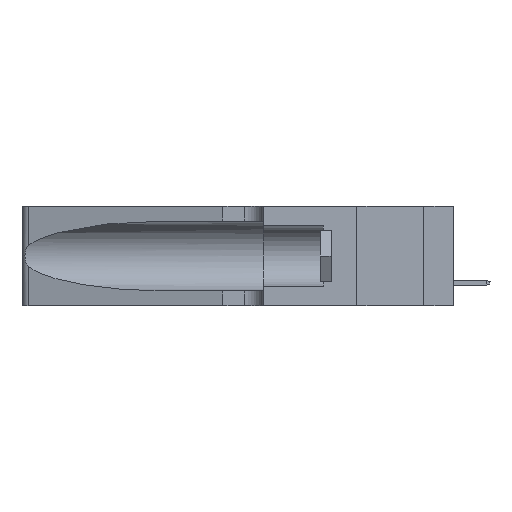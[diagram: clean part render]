
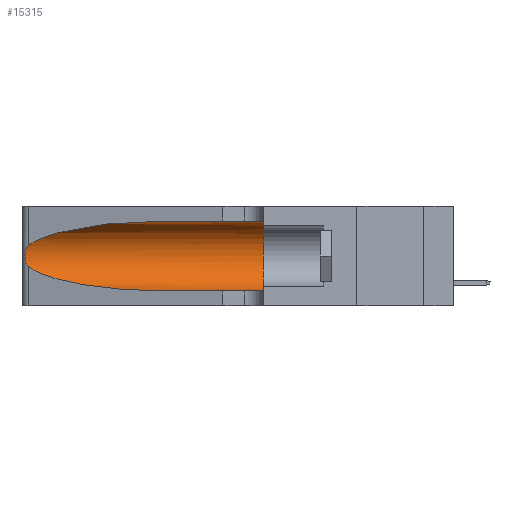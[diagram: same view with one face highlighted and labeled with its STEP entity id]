
A CAD part, left-side view. The second image highlights one B-rep face of the part: STEP entity #15315.
In plain terms, the highlighted cylindrical face has radius 3.308 mm (diameter 6.617 mm), a partial arc.
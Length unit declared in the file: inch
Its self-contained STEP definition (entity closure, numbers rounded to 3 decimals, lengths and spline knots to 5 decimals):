
#363 = EDGE_CURVE ( 'NONE', #2878, #23513, #11433, .T. ) ;
#1574 = CARTESIAN_POINT ( 'NONE',  ( 0.25856, 1.23593, 0.16098 ) ) ;
#1844 = VERTEX_POINT ( 'NONE', #21979 ) ;
#2344 = DIRECTION ( 'NONE',  ( 0., 1., 0. ) ) ;
#2723 = VERTEX_POINT ( 'NONE', #18269 ) ;
#2774 = CARTESIAN_POINT ( 'NONE',  ( 0.1305, 0.35, 0.185 ) ) ;
#2878 = VERTEX_POINT ( 'NONE', #11497 ) ;
#3620 = EDGE_CURVE ( 'NONE', #1844, #23513, #6035, .T. ) ;
#3832 = CARTESIAN_POINT ( 'NONE',  ( 0.25787, 1.23484, 0.2124 ) ) ;
#3941 = VERTEX_POINT ( 'NONE', #9408 ) ;
#4135 = ORIENTED_EDGE ( 'NONE', *, *, #26418, .T. ) ;
#4533 = LINE ( 'NONE', #20291, #17077 ) ;
#4719 = VERTEX_POINT ( 'NONE', #18321 ) ;
#4834 =( BOUNDED_CURVE ( )  B_SPLINE_CURVE ( 3, ( #23729, #9476, #16378, #16237 ),
 .UNSPECIFIED., .F., .T. ) 
 B_SPLINE_CURVE_WITH_KNOTS ( ( 4, 4 ),
 ( 1.5708, 2.84003 ),
 .UNSPECIFIED. ) 
 CURVE ( )  GEOMETRIC_REPRESENTATION_ITEM ( )  RATIONAL_B_SPLINE_CURVE ( ( 1., 0.87, 0.87, 1. ) ) 
 REPRESENTATION_ITEM ( '' )  );
#6035 = LINE ( 'NONE', #15182, #9182 ) ;
#6378 = CARTESIAN_POINT ( 'NONE',  ( 0.25487, 1.22718, 0.14631 ) ) ;
#6846 = EDGE_LOOP ( 'NONE', ( #17508, #28582, #4135, #7560, #24842, #8613 ) ) ;
#7560 = ORIENTED_EDGE ( 'NONE', *, *, #3620, .T. ) ;
#7723 = DIRECTION ( 'NONE',  ( 0., 0., -1. ) ) ;
#8321 = CARTESIAN_POINT ( 'NONE',  ( 0.26075, 1.23896, 0.178 ) ) ;
#8613 = ORIENTED_EDGE ( 'NONE', *, *, #19856, .F. ) ;
#8616 = CARTESIAN_POINT ( 'NONE',  ( 0.26017, 1.23833, 0.17102 ) ) ;
#9182 = VECTOR ( 'NONE', #24656, 39.37008 ) ;
#9408 = CARTESIAN_POINT ( 'NONE',  ( 0.25487, 1.22718, 0.22369 ) ) ;
#9476 = CARTESIAN_POINT ( 'NONE',  ( 0.18966, 0.96281, 0.31525 ) ) ;
#9521 = DIRECTION ( 'NONE',  ( 0., 0., 1. ) ) ;
#9732 = AXIS2_PLACEMENT_3D ( 'NONE', #21690, #19577, #7723 ) ;
#10725 = CARTESIAN_POINT ( 'NONE',  ( 0.25555, 1.22993, 0.14849 ) ) ;
#10987 = CARTESIAN_POINT ( 'NONE',  ( 0.18966, 0.96281, 0.05475 ) ) ;
#11289 = CARTESIAN_POINT ( 'NONE',  ( 0.25487, 1.22718, 0.14631 ) ) ;
#11433 = CIRCLE ( 'NONE', #21479, 0.13025 ) ;
#11497 = CARTESIAN_POINT ( 'NONE',  ( 0.1305, 0.35, 0.31525 ) ) ;
#12967 = CARTESIAN_POINT ( 'NONE',  ( 0.26075, 1.23896, 0.19203 ) ) ;
#13117 = CARTESIAN_POINT ( 'NONE',  ( 0.25854, 1.2359, 0.20912 ) ) ;
#13267 = CARTESIAN_POINT ( 'NONE',  ( 0.26018, 1.23835, 0.19895 ) ) ;
#13670 = DIRECTION ( 'NONE',  ( 0., -1., 0. ) ) ;
#14471 = FACE_OUTER_BOUND ( 'NONE', #6846, .T. ) ;
#14772 = CYLINDRICAL_SURFACE ( 'NONE', #9732, 0.13025 ) ;
#14998 =( BOUNDED_CURVE ( )  B_SPLINE_CURVE ( 3, ( #11289, #25112, #10987, #20154 ),
 .UNSPECIFIED., .F., .T. ) 
 B_SPLINE_CURVE_WITH_KNOTS ( ( 4, 4 ),
 ( 3.44316, 4.71239 ),
 .UNSPECIFIED. ) 
 CURVE ( )  GEOMETRIC_REPRESENTATION_ITEM ( )  RATIONAL_B_SPLINE_CURVE ( ( 1., 0.87, 0.87, 1. ) ) 
 REPRESENTATION_ITEM ( '' )  );
#15182 = CARTESIAN_POINT ( 'NONE',  ( 0.1305, 1.61858, 0.05475 ) ) ;
#15315 = ADVANCED_FACE ( 'NONE', ( #14471 ), #14772, .F. ) ;
#15520 = EDGE_CURVE ( 'NONE', #3941, #4719, #24149, .T. ) ;
#16237 = CARTESIAN_POINT ( 'NONE',  ( 0.25487, 1.22718, 0.22369 ) ) ;
#16378 = CARTESIAN_POINT ( 'NONE',  ( 0.2373, 1.15595, 0.28018 ) ) ;
#17077 = VECTOR ( 'NONE', #13670, 39.37008 ) ;
#17493 = CARTESIAN_POINT ( 'NONE',  ( 0.25789, 1.23486, 0.15765 ) ) ;
#17508 = ORIENTED_EDGE ( 'NONE', *, *, #21508, .T. ) ;
#18269 = CARTESIAN_POINT ( 'NONE',  ( 0.1305, 0.72297, 0.31525 ) ) ;
#18321 = CARTESIAN_POINT ( 'NONE',  ( 0.25487, 1.22718, 0.14631 ) ) ;
#19577 = DIRECTION ( 'NONE',  ( 0., -1., 0. ) ) ;
#19856 = EDGE_CURVE ( 'NONE', #2723, #2878, #4533, .T. ) ;
#20154 = CARTESIAN_POINT ( 'NONE',  ( 0.1305, 0.72297, 0.05475 ) ) ;
#20291 = CARTESIAN_POINT ( 'NONE',  ( 0.1305, 1.61858, 0.31525 ) ) ;
#21479 = AXIS2_PLACEMENT_3D ( 'NONE', #2774, #2344, #9521 ) ;
#21508 = EDGE_CURVE ( 'NONE', #2723, #3941, #4834, .T. ) ;
#21690 = CARTESIAN_POINT ( 'NONE',  ( 0.1305, 1.61858, 0.185 ) ) ;
#21979 = CARTESIAN_POINT ( 'NONE',  ( 0.1305, 0.72297, 0.05475 ) ) ;
#23513 = VERTEX_POINT ( 'NONE', #26846 ) ;
#23729 = CARTESIAN_POINT ( 'NONE',  ( 0.1305, 0.72297, 0.31525 ) ) ;
#24149 = B_SPLINE_CURVE_WITH_KNOTS ( 'NONE', 3,
 ( #28897, #29347, #24543, #3832, #13117, #13267, #12967, #8321, #8616, #1574, #17493, #26935, #10725, #6378 ),
 .UNSPECIFIED., .F., .F.,
 ( 4, 2, 2, 2, 2, 2, 4 ),
 ( 0., 0.00027, 0.00053, 0.00107, 0.0016, 0.00187, 0.00214 ),
 .UNSPECIFIED. ) ;
#24543 = CARTESIAN_POINT ( 'NONE',  ( 0.25639, 1.23184, 0.21858 ) ) ;
#24656 = DIRECTION ( 'NONE',  ( 0., -1., 0. ) ) ;
#24842 = ORIENTED_EDGE ( 'NONE', *, *, #363, .F. ) ;
#25112 = CARTESIAN_POINT ( 'NONE',  ( 0.2373, 1.15595, 0.08982 ) ) ;
#26418 = EDGE_CURVE ( 'NONE', #4719, #1844, #14998, .T. ) ;
#26846 = CARTESIAN_POINT ( 'NONE',  ( 0.1305, 0.35, 0.05475 ) ) ;
#26935 = CARTESIAN_POINT ( 'NONE',  ( 0.25639, 1.23186, 0.15144 ) ) ;
#28582 = ORIENTED_EDGE ( 'NONE', *, *, #15520, .T. ) ;
#28897 = CARTESIAN_POINT ( 'NONE',  ( 0.25487, 1.22718, 0.22369 ) ) ;
#29347 = CARTESIAN_POINT ( 'NONE',  ( 0.25555, 1.22994, 0.2215 ) ) ;
